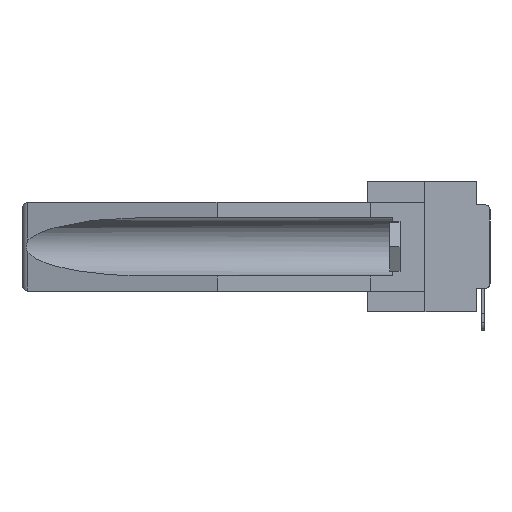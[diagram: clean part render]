
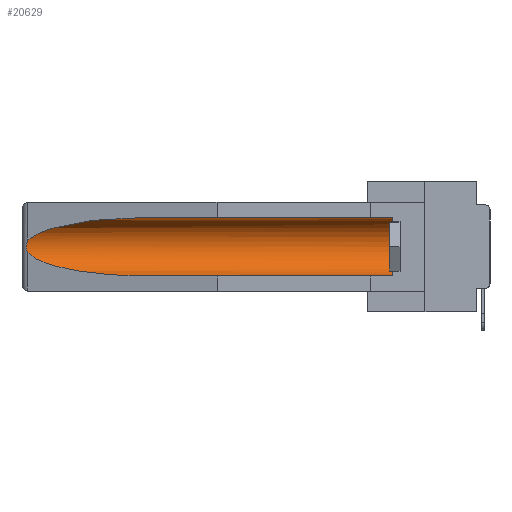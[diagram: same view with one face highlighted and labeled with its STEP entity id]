
A CAD part, left-side view. The second image highlights one B-rep face of the part: STEP entity #20629.
In plain terms, the highlighted cylindrical face has radius 2.857 mm (diameter 5.715 mm), a partial arc.
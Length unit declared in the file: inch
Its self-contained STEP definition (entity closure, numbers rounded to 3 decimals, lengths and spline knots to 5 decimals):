
#593 = VERTEX_POINT ( 'NONE', #4302 ) ;
#719 = VERTEX_POINT ( 'NONE', #12425 ) ;
#2225 = ORIENTED_EDGE ( 'NONE', *, *, #11094, .F. ) ;
#2535 = CARTESIAN_POINT ( 'NONE',  ( 0.2673, 1.53269, -0.17917 ) ) ;
#2579 = EDGE_CURVE ( 'NONE', #593, #29205, #5295, .T. ) ;
#2831 = EDGE_CURVE ( 'NONE', #29205, #719, #6467, .T. ) ;
#4302 = CARTESIAN_POINT ( 'NONE',  ( 0.155, 0.126, -0.284 ) ) ;
#4728 =( BOUNDED_CURVE ( )  B_SPLINE_CURVE ( 3, ( #24339, #11427, #13813, #32054 ),
 .UNSPECIFIED., .F., .F. ) 
 B_SPLINE_CURVE_WITH_KNOTS ( ( 4, 4 ),
 ( 0.1948, 1.5708 ),
 .UNSPECIFIED. ) 
 CURVE ( )  GEOMETRIC_REPRESENTATION_ITEM ( )  RATIONAL_B_SPLINE_CURVE ( ( 1., 0.848, 0.848, 1. ) ) 
 REPRESENTATION_ITEM ( '' )  );
#5274 = CARTESIAN_POINT ( 'NONE',  ( 0.26537, 1.52718, -0.19328 ) ) ;
#5295 = CIRCLE ( 'NONE', #8688, 0.1125 ) ;
#6193 = CARTESIAN_POINT ( 'NONE',  ( 0.155, -0.30754, -0.059 ) ) ;
#6336 = ORIENTED_EDGE ( 'NONE', *, *, #19598, .T. ) ;
#6359 = CARTESIAN_POINT ( 'NONE',  ( 0.21114, 1.30732, -0.059 ) ) ;
#6415 = DIRECTION ( 'NONE',  ( 0., 1., 0. ) ) ;
#6467 = LINE ( 'NONE', #6193, #19013 ) ;
#7734 = CARTESIAN_POINT ( 'NONE',  ( 0.26655, 1.53094, -0.18657 ) ) ;
#8688 = AXIS2_PLACEMENT_3D ( 'NONE', #33072, #9618, #20404 ) ;
#9618 = DIRECTION ( 'NONE',  ( 0., -1., 0. ) ) ;
#10002 = CARTESIAN_POINT ( 'NONE',  ( 0.26537, 1.52718, -0.14972 ) ) ;
#11053 = ORIENTED_EDGE ( 'NONE', *, *, #2831, .T. ) ;
#11094 = EDGE_CURVE ( 'NONE', #593, #23066, #17372, .T. ) ;
#11398 = EDGE_LOOP ( 'NONE', ( #18881, #20841, #6336, #2225, #25878, #11053 ) ) ;
#11427 = CARTESIAN_POINT ( 'NONE',  ( 0.25451, 1.48313, -0.24835 ) ) ;
#11944 = CARTESIAN_POINT ( 'NONE',  ( 0.26537, 1.52718, -0.14972 ) ) ;
#12425 = CARTESIAN_POINT ( 'NONE',  ( 0.155, 1.07973, -0.059 ) ) ;
#13050 = CARTESIAN_POINT ( 'NONE',  ( 0.26597, 1.52961, -0.15275 ) ) ;
#13514 = FACE_OUTER_BOUND ( 'NONE', #11398, .T. ) ;
#13517 = DIRECTION ( 'NONE',  ( 0., 1., 0. ) ) ;
#13813 = CARTESIAN_POINT ( 'NONE',  ( 0.21114, 1.30732, -0.284 ) ) ;
#15320 = CARTESIAN_POINT ( 'NONE',  ( 0.2675, 1.53308, -0.16763 ) ) ;
#15520 = CARTESIAN_POINT ( 'NONE',  ( 0.2675, 1.53308, -0.17534 ) ) ;
#17345 = CARTESIAN_POINT ( 'NONE',  ( 0.26537, 1.52718, -0.19328 ) ) ;
#17372 = LINE ( 'NONE', #23708, #22258 ) ;
#17911 = CARTESIAN_POINT ( 'NONE',  ( 0.2673, 1.5327, -0.16383 ) ) ;
#18138 = EDGE_CURVE ( 'NONE', #31191, #20757, #32727, .T. ) ;
#18365 = CYLINDRICAL_SURFACE ( 'NONE', #23836, 0.1125 ) ;
#18881 = ORIENTED_EDGE ( 'NONE', *, *, #28706, .T. ) ;
#19013 = VECTOR ( 'NONE', #22000, 39.37008 ) ;
#19237 = CARTESIAN_POINT ( 'NONE',  ( 0.26537, 1.52718, -0.14972 ) ) ;
#19524 = CARTESIAN_POINT ( 'NONE',  ( 0.155, -0.30754, -0.1715 ) ) ;
#19598 = EDGE_CURVE ( 'NONE', #20757, #23066, #4728, .T. ) ;
#20404 = DIRECTION ( 'NONE',  ( 0., 0., 1. ) ) ;
#20629 = ADVANCED_FACE ( 'NONE', ( #13514 ), #18365, .F. ) ;
#20757 = VERTEX_POINT ( 'NONE', #17345 ) ;
#20841 = ORIENTED_EDGE ( 'NONE', *, *, #18138, .T. ) ;
#22000 = DIRECTION ( 'NONE',  ( 0., 1., 0. ) ) ;
#22258 = VECTOR ( 'NONE', #13517, 39.37008 ) ;
#23066 = VERTEX_POINT ( 'NONE', #30823 ) ;
#23708 = CARTESIAN_POINT ( 'NONE',  ( 0.155, -0.30754, -0.284 ) ) ;
#23743 = CARTESIAN_POINT ( 'NONE',  ( 0.155, 0.126, -0.059 ) ) ;
#23836 = AXIS2_PLACEMENT_3D ( 'NONE', #19524, #6415, #27080 ) ;
#24339 = CARTESIAN_POINT ( 'NONE',  ( 0.26537, 1.52718, -0.19328 ) ) ;
#25593 = CARTESIAN_POINT ( 'NONE',  ( 0.26654, 1.53092, -0.15636 ) ) ;
#25878 = ORIENTED_EDGE ( 'NONE', *, *, #2579, .T. ) ;
#27080 = DIRECTION ( 'NONE',  ( 0., 0., 1. ) ) ;
#27300 =( BOUNDED_CURVE ( )  B_SPLINE_CURVE ( 3, ( #32386, #6359, #31921, #19237 ),
 .UNSPECIFIED., .F., .F. ) 
 B_SPLINE_CURVE_WITH_KNOTS ( ( 4, 4 ),
 ( 4.71239, 6.08839 ),
 .UNSPECIFIED. ) 
 CURVE ( )  GEOMETRIC_REPRESENTATION_ITEM ( )  RATIONAL_B_SPLINE_CURVE ( ( 1., 0.848, 0.848, 1. ) ) 
 REPRESENTATION_ITEM ( '' )  );
#28706 = EDGE_CURVE ( 'NONE', #719, #31191, #27300, .T. ) ;
#29205 = VERTEX_POINT ( 'NONE', #23743 ) ;
#30823 = CARTESIAN_POINT ( 'NONE',  ( 0.155, 1.07973, -0.284 ) ) ;
#31166 = CARTESIAN_POINT ( 'NONE',  ( 0.26597, 1.5296, -0.19026 ) ) ;
#31191 = VERTEX_POINT ( 'NONE', #11944 ) ;
#31921 = CARTESIAN_POINT ( 'NONE',  ( 0.25451, 1.48313, -0.09465 ) ) ;
#32054 = CARTESIAN_POINT ( 'NONE',  ( 0.155, 1.07973, -0.284 ) ) ;
#32386 = CARTESIAN_POINT ( 'NONE',  ( 0.155, 1.07973, -0.059 ) ) ;
#32727 = B_SPLINE_CURVE_WITH_KNOTS ( 'NONE', 3,
 ( #10002, #13050, #25593, #17911, #15320, #15520, #2535, #7734, #31166, #5274 ),
 .UNSPECIFIED., .F., .F.,
 ( 4, 2, 2, 2, 4 ),
 ( 0., 0.00029, 0.00058, 0.00087, 0.00117 ),
 .UNSPECIFIED. ) ;
#33072 = CARTESIAN_POINT ( 'NONE',  ( 0.155, 0.126, -0.1715 ) ) ;
